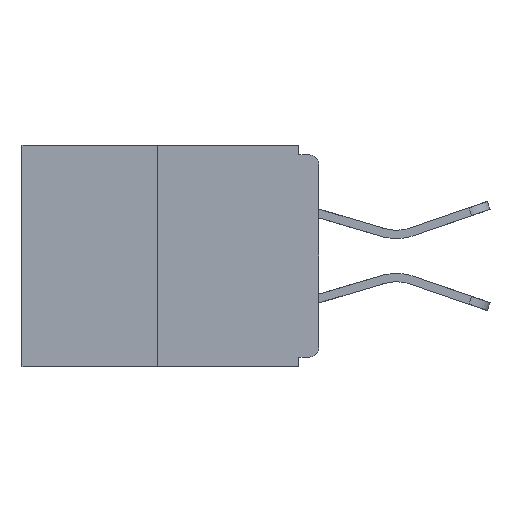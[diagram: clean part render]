
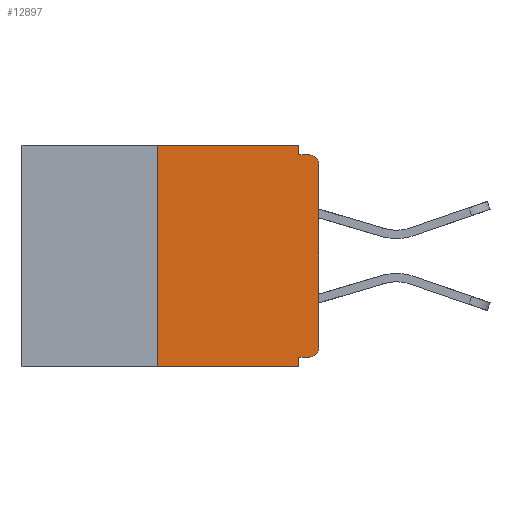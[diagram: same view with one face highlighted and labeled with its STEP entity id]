
A CAD part, left-side view. The second image highlights one B-rep face of the part: STEP entity #12897.
In plain terms, the highlighted planar face has unit normal (-1, 0, 0).
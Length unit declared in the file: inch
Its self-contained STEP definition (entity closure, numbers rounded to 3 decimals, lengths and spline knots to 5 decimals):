
#364 = DIRECTION ( 'NONE',  ( 0., 0., -1. ) ) ;
#775 = VERTEX_POINT ( 'NONE', #11353 ) ;
#797 = CARTESIAN_POINT ( 'NONE',  ( 0., 0.46, 0. ) ) ;
#1227 = DIRECTION ( 'NONE',  ( 0., 0., -1. ) ) ;
#1762 = DIRECTION ( 'NONE',  ( 0., 1., 0. ) ) ;
#2072 = ORIENTED_EDGE ( 'NONE', *, *, #21315, .F. ) ;
#2773 = ORIENTED_EDGE ( 'NONE', *, *, #5895, .T. ) ;
#3174 = CARTESIAN_POINT ( 'NONE',  ( 0., 0.015, -0.03 ) ) ;
#3723 = EDGE_CURVE ( 'NONE', #19146, #11638, #8181, .T. ) ;
#3777 = VERTEX_POINT ( 'NONE', #5844 ) ;
#4781 = EDGE_CURVE ( 'NONE', #17208, #10536, #8127, .T. ) ;
#5303 = CARTESIAN_POINT ( 'NONE',  ( 0., 0.031, -0.328 ) ) ;
#5349 = CARTESIAN_POINT ( 'NONE',  ( 0., 0.031, 0. ) ) ;
#5844 = CARTESIAN_POINT ( 'NONE',  ( 0., 0.031, 0. ) ) ;
#5895 = EDGE_CURVE ( 'NONE', #775, #26911, #17541, .T. ) ;
#6058 = FACE_OUTER_BOUND ( 'NONE', #24149, .T. ) ;
#6807 = ORIENTED_EDGE ( 'NONE', *, *, #3723, .T. ) ;
#7210 = VECTOR ( 'NONE', #1762, 39.37008 ) ;
#7310 = AXIS2_PLACEMENT_3D ( 'NONE', #3174, #24155, #11520 ) ;
#7504 = VECTOR ( 'NONE', #1227, 39.37008 ) ;
#7509 = CARTESIAN_POINT ( 'NONE',  ( 0., 0.25, 0. ) ) ;
#7561 = VECTOR ( 'NONE', #24926, 39.37008 ) ;
#7839 = VERTEX_POINT ( 'NONE', #5303 ) ;
#8061 = DIRECTION ( 'NONE',  ( -1., 0., 0. ) ) ;
#8127 = LINE ( 'NONE', #13180, #9714 ) ;
#8172 = AXIS2_PLACEMENT_3D ( 'NONE', #10134, #8061, #20632 ) ;
#8181 = CIRCLE ( 'NONE', #8172, 0.015 ) ;
#9450 = CARTESIAN_POINT ( 'NONE',  ( 0., 0., -0.313 ) ) ;
#9563 = VECTOR ( 'NONE', #17444, 39.37008 ) ;
#9714 = VECTOR ( 'NONE', #21588, 39.37008 ) ;
#10040 = EDGE_CURVE ( 'NONE', #24385, #26911, #24670, .T. ) ;
#10123 = ORIENTED_EDGE ( 'NONE', *, *, #18222, .F. ) ;
#10134 = CARTESIAN_POINT ( 'NONE',  ( 0., 0.015, -0.313 ) ) ;
#10221 = EDGE_CURVE ( 'NONE', #7839, #10536, #13720, .T. ) ;
#10526 = PLANE ( 'NONE',  #10929 ) ;
#10536 = VERTEX_POINT ( 'NONE', #16809 ) ;
#10617 = DIRECTION ( 'NONE',  ( 1., 0., 0. ) ) ;
#10762 = EDGE_CURVE ( 'NONE', #3777, #24385, #13057, .T. ) ;
#10929 = AXIS2_PLACEMENT_3D ( 'NONE', #25279, #10617, #25376 ) ;
#11248 = ORIENTED_EDGE ( 'NONE', *, *, #4781, .T. ) ;
#11353 = CARTESIAN_POINT ( 'NONE',  ( 0., 0., -0.03 ) ) ;
#11520 = DIRECTION ( 'NONE',  ( 0., 0., -1. ) ) ;
#11638 = VERTEX_POINT ( 'NONE', #9450 ) ;
#12897 = ADVANCED_FACE ( 'NONE', ( #6058 ), #10526, .F. ) ;
#13057 = LINE ( 'NONE', #5349, #7504 ) ;
#13180 = CARTESIAN_POINT ( 'NONE',  ( 0., 0.46, -0.343 ) ) ;
#13560 = ORIENTED_EDGE ( 'NONE', *, *, #10221, .F. ) ;
#13720 = LINE ( 'NONE', #21371, #19690 ) ;
#14257 = EDGE_CURVE ( 'NONE', #11638, #775, #20777, .T. ) ;
#14476 = VERTEX_POINT ( 'NONE', #7509 ) ;
#15592 = LINE ( 'NONE', #23066, #20192 ) ;
#16589 = ORIENTED_EDGE ( 'NONE', *, *, #10762, .F. ) ;
#16732 = LINE ( 'NONE', #20910, #7210 ) ;
#16809 = CARTESIAN_POINT ( 'NONE',  ( 0., 0.031, -0.343 ) ) ;
#17208 = VERTEX_POINT ( 'NONE', #26002 ) ;
#17283 = ORIENTED_EDGE ( 'NONE', *, *, #14257, .T. ) ;
#17444 = DIRECTION ( 'NONE',  ( 0., 0., 1. ) ) ;
#17541 = CIRCLE ( 'NONE', #7310, 0.015 ) ;
#17864 = ORIENTED_EDGE ( 'NONE', *, *, #10040, .F. ) ;
#18097 = VECTOR ( 'NONE', #21987, 39.37008 ) ;
#18222 = EDGE_CURVE ( 'NONE', #17208, #14476, #15592, .T. ) ;
#18801 = DIRECTION ( 'NONE',  ( 0., 0., 1. ) ) ;
#19146 = VERTEX_POINT ( 'NONE', #23848 ) ;
#19690 = VECTOR ( 'NONE', #364, 39.37008 ) ;
#19812 = CARTESIAN_POINT ( 'NONE',  ( 0., 0.031, -0.015 ) ) ;
#20029 = ORIENTED_EDGE ( 'NONE', *, *, #22909, .F. ) ;
#20192 = VECTOR ( 'NONE', #18801, 39.37008 ) ;
#20632 = DIRECTION ( 'NONE',  ( 0., 0., -1. ) ) ;
#20777 = LINE ( 'NONE', #23207, #9563 ) ;
#20910 = CARTESIAN_POINT ( 'NONE',  ( 0., 0., -0.328 ) ) ;
#21315 = EDGE_CURVE ( 'NONE', #19146, #7839, #16732, .T. ) ;
#21371 = CARTESIAN_POINT ( 'NONE',  ( 0., 0.031, -0.343 ) ) ;
#21588 = DIRECTION ( 'NONE',  ( 0., -1., 0. ) ) ;
#21987 = DIRECTION ( 'NONE',  ( 0., -1., 0. ) ) ;
#22223 = CARTESIAN_POINT ( 'NONE',  ( 0., 0.015, -0.015 ) ) ;
#22909 = EDGE_CURVE ( 'NONE', #14476, #3777, #25399, .T. ) ;
#23066 = CARTESIAN_POINT ( 'NONE',  ( 0., 0.25, 0. ) ) ;
#23089 = CARTESIAN_POINT ( 'NONE',  ( 0., 0., -0.015 ) ) ;
#23207 = CARTESIAN_POINT ( 'NONE',  ( 0., 0., 0. ) ) ;
#23848 = CARTESIAN_POINT ( 'NONE',  ( 0., 0.015, -0.328 ) ) ;
#24149 = EDGE_LOOP ( 'NONE', ( #20029, #10123, #11248, #13560, #2072, #6807, #17283, #2773, #17864, #16589 ) ) ;
#24155 = DIRECTION ( 'NONE',  ( -1., 0., 0. ) ) ;
#24385 = VERTEX_POINT ( 'NONE', #19812 ) ;
#24670 = LINE ( 'NONE', #23089, #7561 ) ;
#24926 = DIRECTION ( 'NONE',  ( 0., -1., 0. ) ) ;
#25279 = CARTESIAN_POINT ( 'NONE',  ( 0., 0.46, 0. ) ) ;
#25376 = DIRECTION ( 'NONE',  ( 0., 0., -1. ) ) ;
#25399 = LINE ( 'NONE', #797, #18097 ) ;
#26002 = CARTESIAN_POINT ( 'NONE',  ( 0., 0.25, -0.343 ) ) ;
#26911 = VERTEX_POINT ( 'NONE', #22223 ) ;
